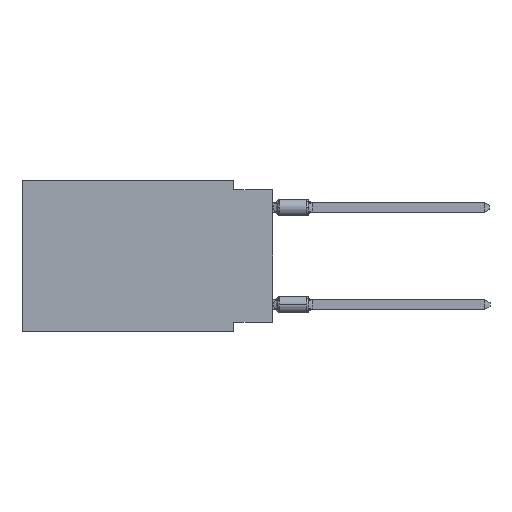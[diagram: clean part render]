
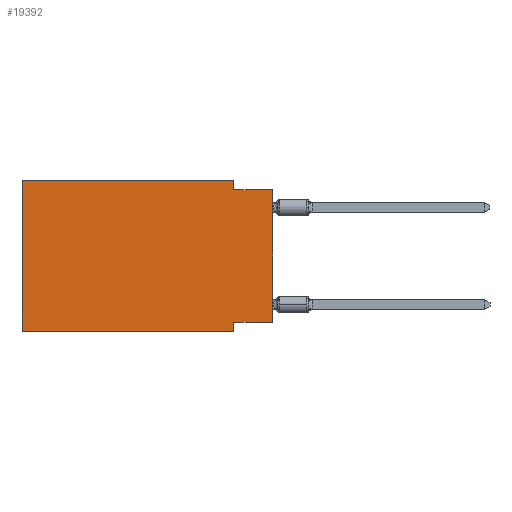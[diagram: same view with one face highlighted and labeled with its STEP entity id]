
A CAD part, left-side view. The second image highlights one B-rep face of the part: STEP entity #19392.
In plain terms, the highlighted planar face has unit normal (-1, 0, 0).
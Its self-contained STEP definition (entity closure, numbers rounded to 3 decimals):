
#308 = VERTEX_POINT ( 'NONE', #14082 ) ;
#359 = ORIENTED_EDGE ( 'NONE', *, *, #17854, .F. ) ;
#609 = CARTESIAN_POINT ( 'NONE',  ( 0., 16.383, 0. ) ) ;
#728 = CARTESIAN_POINT ( 'NONE',  ( 0., 2.54, -9.271 ) ) ;
#1208 = VERTEX_POINT ( 'NONE', #17437 ) ;
#1629 = ORIENTED_EDGE ( 'NONE', *, *, #11902, .T. ) ;
#1985 = LINE ( 'NONE', #4065, #20980 ) ;
#2366 = EDGE_CURVE ( 'NONE', #20010, #2731, #9256, .T. ) ;
#2475 = EDGE_CURVE ( 'NONE', #1208, #9903, #15379, .T. ) ;
#2687 = EDGE_LOOP ( 'NONE', ( #23439, #22269, #11114, #359, #21687, #1629, #23648, #15667 ) ) ;
#2731 = VERTEX_POINT ( 'NONE', #728 ) ;
#3125 = DIRECTION ( 'NONE',  ( 0., -1., 0. ) ) ;
#3802 = DIRECTION ( 'NONE',  ( 1., 0., 0. ) ) ;
#3813 = CARTESIAN_POINT ( 'NONE',  ( 0., 2.54, -0.635 ) ) ;
#4065 = CARTESIAN_POINT ( 'NONE',  ( 0., 2.54, 0. ) ) ;
#4881 = LINE ( 'NONE', #4999, #22868 ) ;
#4999 = CARTESIAN_POINT ( 'NONE',  ( 0., 16.383, -9.906 ) ) ;
#5195 = LINE ( 'NONE', #8957, #5552 ) ;
#5463 = CARTESIAN_POINT ( 'NONE',  ( 0., 0., -0.635 ) ) ;
#5552 = VECTOR ( 'NONE', #3125, 1000. ) ;
#5574 = VECTOR ( 'NONE', #5857, 1000. ) ;
#5716 = DIRECTION ( 'NONE',  ( 0., -1., 0. ) ) ;
#5857 = DIRECTION ( 'NONE',  ( 0., 0., 1. ) ) ;
#6156 = VECTOR ( 'NONE', #17057, 1000. ) ;
#7077 = CARTESIAN_POINT ( 'NONE',  ( 0., 0., -9.271 ) ) ;
#7721 = CARTESIAN_POINT ( 'NONE',  ( 0., 16.383, 0. ) ) ;
#7905 = CARTESIAN_POINT ( 'NONE',  ( 0., 0., 0. ) ) ;
#7921 = VECTOR ( 'NONE', #10842, 1000. ) ;
#8036 = DIRECTION ( 'NONE',  ( 0., 0., -1. ) ) ;
#8296 = CARTESIAN_POINT ( 'NONE',  ( 0., 0., -9.271 ) ) ;
#8957 = CARTESIAN_POINT ( 'NONE',  ( 0., 16.383, 0. ) ) ;
#9256 = LINE ( 'NONE', #7077, #7921 ) ;
#9903 = VERTEX_POINT ( 'NONE', #7721 ) ;
#10330 = EDGE_CURVE ( 'NONE', #20010, #308, #15108, .T. ) ;
#10842 = DIRECTION ( 'NONE',  ( 0., 1., 0. ) ) ;
#11114 = ORIENTED_EDGE ( 'NONE', *, *, #23267, .F. ) ;
#11902 = EDGE_CURVE ( 'NONE', #1208, #14942, #4881, .T. ) ;
#12058 = EDGE_CURVE ( 'NONE', #18347, #308, #22208, .T. ) ;
#13329 = EDGE_CURVE ( 'NONE', #2731, #14942, #13909, .T. ) ;
#13425 = AXIS2_PLACEMENT_3D ( 'NONE', #16865, #3802, #20795 ) ;
#13504 = FACE_OUTER_BOUND ( 'NONE', #2687, .T. ) ;
#13909 = LINE ( 'NONE', #22839, #18414 ) ;
#14082 = CARTESIAN_POINT ( 'NONE',  ( 0., 0., -0.635 ) ) ;
#14942 = VERTEX_POINT ( 'NONE', #20029 ) ;
#15108 = LINE ( 'NONE', #7905, #6156 ) ;
#15205 = CARTESIAN_POINT ( 'NONE',  ( 0., 2.54, 0. ) ) ;
#15379 = LINE ( 'NONE', #609, #5574 ) ;
#15667 = ORIENTED_EDGE ( 'NONE', *, *, #2366, .F. ) ;
#16865 = CARTESIAN_POINT ( 'NONE',  ( 0., 16.383, 0. ) ) ;
#17057 = DIRECTION ( 'NONE',  ( 0., 0., 1. ) ) ;
#17437 = CARTESIAN_POINT ( 'NONE',  ( 0., 16.383, -9.906 ) ) ;
#17854 = EDGE_CURVE ( 'NONE', #9903, #19242, #5195, .T. ) ;
#18347 = VERTEX_POINT ( 'NONE', #3813 ) ;
#18414 = VECTOR ( 'NONE', #8036, 1000. ) ;
#19242 = VERTEX_POINT ( 'NONE', #15205 ) ;
#19392 = ADVANCED_FACE ( 'NONE', ( #13504 ), #20969, .F. ) ;
#20010 = VERTEX_POINT ( 'NONE', #8296 ) ;
#20027 = DIRECTION ( 'NONE',  ( 0., -1., 0. ) ) ;
#20029 = CARTESIAN_POINT ( 'NONE',  ( 0., 2.54, -9.906 ) ) ;
#20795 = DIRECTION ( 'NONE',  ( 0., 0., -1. ) ) ;
#20969 = PLANE ( 'NONE',  #13425 ) ;
#20980 = VECTOR ( 'NONE', #21060, 1000. ) ;
#21060 = DIRECTION ( 'NONE',  ( 0., 0., -1. ) ) ;
#21128 = VECTOR ( 'NONE', #5716, 1000. ) ;
#21687 = ORIENTED_EDGE ( 'NONE', *, *, #2475, .F. ) ;
#22208 = LINE ( 'NONE', #5463, #21128 ) ;
#22269 = ORIENTED_EDGE ( 'NONE', *, *, #12058, .F. ) ;
#22839 = CARTESIAN_POINT ( 'NONE',  ( 0., 2.54, -9.906 ) ) ;
#22868 = VECTOR ( 'NONE', #20027, 1000. ) ;
#23267 = EDGE_CURVE ( 'NONE', #19242, #18347, #1985, .T. ) ;
#23439 = ORIENTED_EDGE ( 'NONE', *, *, #10330, .T. ) ;
#23648 = ORIENTED_EDGE ( 'NONE', *, *, #13329, .F. ) ;
